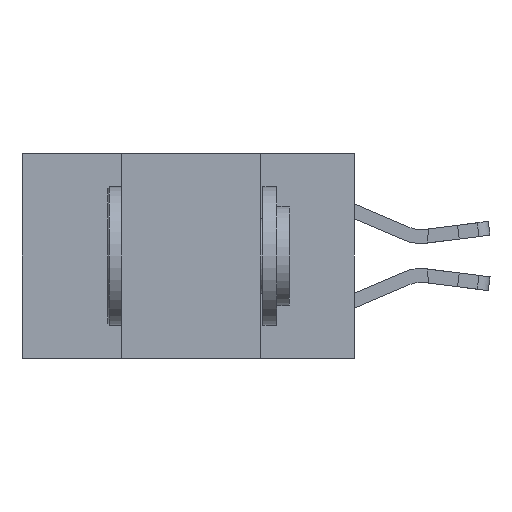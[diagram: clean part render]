
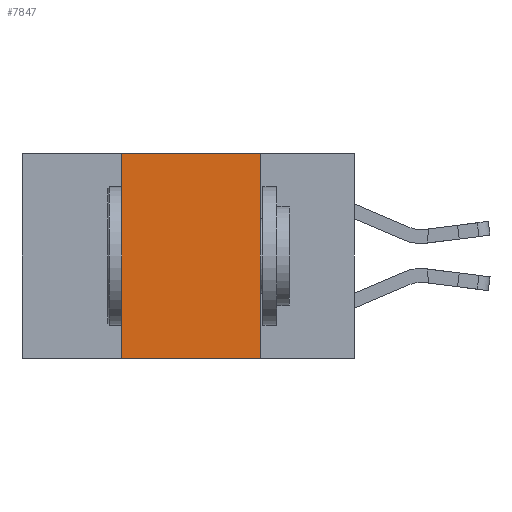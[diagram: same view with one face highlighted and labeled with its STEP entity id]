
A CAD part, left-side view. The second image highlights one B-rep face of the part: STEP entity #7847.
In plain terms, the highlighted planar face has unit normal (-1, 0, 0).
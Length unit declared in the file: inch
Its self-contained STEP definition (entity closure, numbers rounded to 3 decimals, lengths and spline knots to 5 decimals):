
#326 = CARTESIAN_POINT ( 'NONE',  ( 0., 0.17, -0.37 ) ) ;
#1668 = EDGE_CURVE ( 'NONE', #5764, #5686, #5641, .T. ) ;
#1887 = DIRECTION ( 'NONE',  ( 0., -1., 0. ) ) ;
#2381 = VECTOR ( 'NONE', #19126, 39.37008 ) ;
#2623 = EDGE_CURVE ( 'NONE', #11047, #3755, #15333, .T. ) ;
#2886 = ORIENTED_EDGE ( 'NONE', *, *, #1668, .F. ) ;
#3113 = EDGE_LOOP ( 'NONE', ( #19142, #10766, #2886, #11873 ) ) ;
#3512 = EDGE_CURVE ( 'NONE', #5764, #3755, #15059, .T. ) ;
#3755 = VERTEX_POINT ( 'NONE', #326 ) ;
#4125 = AXIS2_PLACEMENT_3D ( 'NONE', #7702, #18662, #7499 ) ;
#5543 = EDGE_CURVE ( 'NONE', #5686, #11047, #10355, .T. ) ;
#5641 = LINE ( 'NONE', #14537, #15346 ) ;
#5686 = VERTEX_POINT ( 'NONE', #6963 ) ;
#5764 = VERTEX_POINT ( 'NONE', #10274 ) ;
#6096 = CARTESIAN_POINT ( 'NONE',  ( 0., 0.17, 0. ) ) ;
#6963 = CARTESIAN_POINT ( 'NONE',  ( 0., 0.42, 0. ) ) ;
#7499 = DIRECTION ( 'NONE',  ( 0., 0., -1. ) ) ;
#7702 = CARTESIAN_POINT ( 'NONE',  ( 0., 0.6, 0. ) ) ;
#7847 = ADVANCED_FACE ( 'NONE', ( #11422 ), #12070, .F. ) ;
#7971 = CARTESIAN_POINT ( 'NONE',  ( 0., 0.6, 0. ) ) ;
#10274 = CARTESIAN_POINT ( 'NONE',  ( 0., 0.42, -0.37 ) ) ;
#10355 = LINE ( 'NONE', #7971, #2381 ) ;
#10766 = ORIENTED_EDGE ( 'NONE', *, *, #5543, .F. ) ;
#11047 = VERTEX_POINT ( 'NONE', #19409 ) ;
#11122 = CARTESIAN_POINT ( 'NONE',  ( 0., 0.6, -0.37 ) ) ;
#11422 = FACE_OUTER_BOUND ( 'NONE', #3113, .T. ) ;
#11873 = ORIENTED_EDGE ( 'NONE', *, *, #3512, .T. ) ;
#12070 = PLANE ( 'NONE',  #4125 ) ;
#14537 = CARTESIAN_POINT ( 'NONE',  ( 0., 0.42, 0. ) ) ;
#15059 = LINE ( 'NONE', #11122, #18696 ) ;
#15333 = LINE ( 'NONE', #6096, #16811 ) ;
#15346 = VECTOR ( 'NONE', #18957, 39.37008 ) ;
#16811 = VECTOR ( 'NONE', #18640, 39.37008 ) ;
#18640 = DIRECTION ( 'NONE',  ( 0., 0., -1. ) ) ;
#18662 = DIRECTION ( 'NONE',  ( 1., 0., 0. ) ) ;
#18696 = VECTOR ( 'NONE', #1887, 39.37008 ) ;
#18957 = DIRECTION ( 'NONE',  ( 0., 0., 1. ) ) ;
#19126 = DIRECTION ( 'NONE',  ( 0., -1., 0. ) ) ;
#19142 = ORIENTED_EDGE ( 'NONE', *, *, #2623, .F. ) ;
#19409 = CARTESIAN_POINT ( 'NONE',  ( 0., 0.17, 0. ) ) ;
